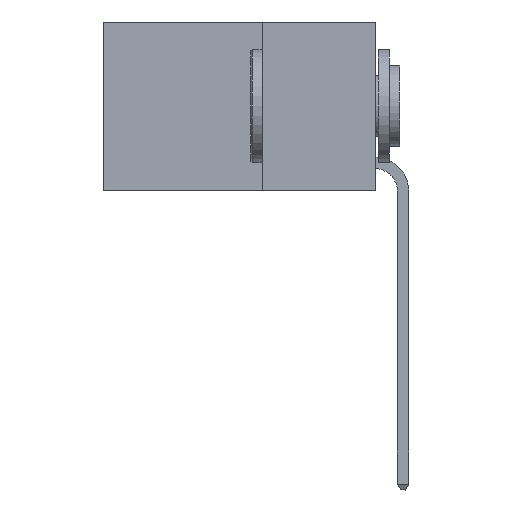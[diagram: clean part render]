
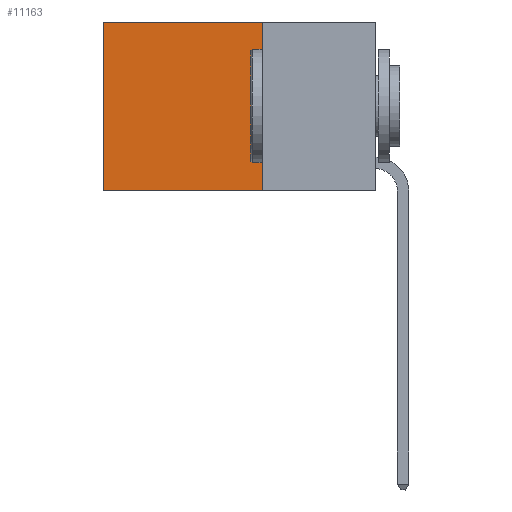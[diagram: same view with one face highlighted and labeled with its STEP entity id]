
A CAD part, left-side view. The second image highlights one B-rep face of the part: STEP entity #11163.
In plain terms, the highlighted planar face has unit normal (-1, 0, 0).
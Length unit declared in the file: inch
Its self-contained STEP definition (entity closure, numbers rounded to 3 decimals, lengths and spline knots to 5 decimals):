
#482 = FACE_OUTER_BOUND ( 'NONE', #10756, .T. ) ;
#888 = CARTESIAN_POINT ( 'NONE',  ( 0.2625, 0.6, 0. ) ) ;
#1297 = ORIENTED_EDGE ( 'NONE', *, *, #16399, .F. ) ;
#1312 = VERTEX_POINT ( 'NONE', #12678 ) ;
#1319 = EDGE_CURVE ( 'NONE', #7430, #16366, #2606, .T. ) ;
#1533 = DIRECTION ( 'NONE',  ( 0., 0., -1. ) ) ;
#1609 = EDGE_CURVE ( 'NONE', #8378, #16366, #10091, .T. ) ;
#2397 = CARTESIAN_POINT ( 'NONE',  ( 0.2625, 0.25, -0.37 ) ) ;
#2606 = LINE ( 'NONE', #11003, #3124 ) ;
#3124 = VECTOR ( 'NONE', #9054, 39.37008 ) ;
#4128 = ORIENTED_EDGE ( 'NONE', *, *, #1319, .T. ) ;
#4260 = CARTESIAN_POINT ( 'NONE',  ( 0.2625, 0.25, 0. ) ) ;
#4833 = CARTESIAN_POINT ( 'NONE',  ( 0.2625, 0.25, -0.37 ) ) ;
#5852 = VECTOR ( 'NONE', #1533, 39.37008 ) ;
#5888 = DIRECTION ( 'NONE',  ( 1., 0., 0. ) ) ;
#6350 = CARTESIAN_POINT ( 'NONE',  ( 0.2625, 0.25, 0. ) ) ;
#6528 = VECTOR ( 'NONE', #18577, 39.37008 ) ;
#6632 = VECTOR ( 'NONE', #16539, 39.37008 ) ;
#7019 = LINE ( 'NONE', #9150, #6528 ) ;
#7430 = VERTEX_POINT ( 'NONE', #888 ) ;
#8378 = VERTEX_POINT ( 'NONE', #4833 ) ;
#9054 = DIRECTION ( 'NONE',  ( 0., 0., -1. ) ) ;
#9150 = CARTESIAN_POINT ( 'NONE',  ( 0.2625, 0.25, 0. ) ) ;
#10091 = LINE ( 'NONE', #2397, #6632 ) ;
#10756 = EDGE_LOOP ( 'NONE', ( #4128, #16470, #1297, #17913 ) ) ;
#11003 = CARTESIAN_POINT ( 'NONE',  ( 0.2625, 0.6, 0. ) ) ;
#11163 = ADVANCED_FACE ( 'NONE', ( #482 ), #15319, .F. ) ;
#12545 = CARTESIAN_POINT ( 'NONE',  ( 0.2625, 0.6, -0.37 ) ) ;
#12678 = CARTESIAN_POINT ( 'NONE',  ( 0.2625, 0.25, 0. ) ) ;
#15319 = PLANE ( 'NONE',  #16457 ) ;
#16366 = VERTEX_POINT ( 'NONE', #12545 ) ;
#16399 = EDGE_CURVE ( 'NONE', #1312, #8378, #18397, .T. ) ;
#16457 = AXIS2_PLACEMENT_3D ( 'NONE', #4260, #5888, #16900 ) ;
#16470 = ORIENTED_EDGE ( 'NONE', *, *, #1609, .F. ) ;
#16539 = DIRECTION ( 'NONE',  ( 0., 1., 0. ) ) ;
#16900 = DIRECTION ( 'NONE',  ( 0., 0., -1. ) ) ;
#17913 = ORIENTED_EDGE ( 'NONE', *, *, #18133, .T. ) ;
#18133 = EDGE_CURVE ( 'NONE', #1312, #7430, #7019, .T. ) ;
#18397 = LINE ( 'NONE', #6350, #5852 ) ;
#18577 = DIRECTION ( 'NONE',  ( 0., 1., 0. ) ) ;
